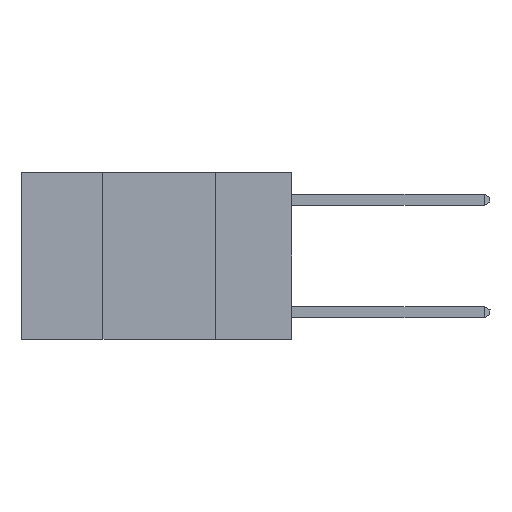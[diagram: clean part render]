
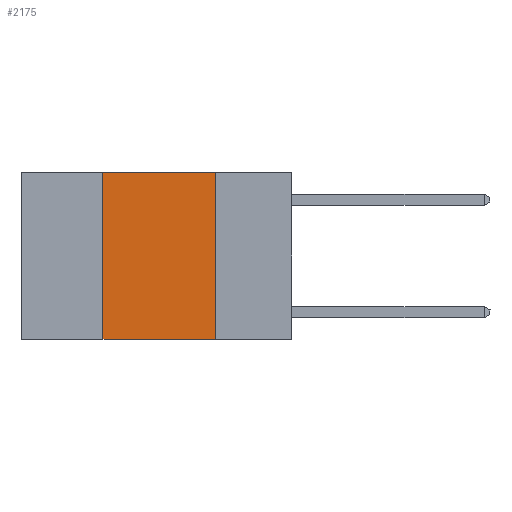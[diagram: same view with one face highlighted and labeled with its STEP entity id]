
A CAD part, left-side view. The second image highlights one B-rep face of the part: STEP entity #2175.
In plain terms, the highlighted planar face has unit normal (-1, 0, 0).
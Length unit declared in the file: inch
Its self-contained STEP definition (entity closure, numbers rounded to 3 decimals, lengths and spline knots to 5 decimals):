
#514 = PLANE ( 'NONE',  #21172 ) ;
#680 = VECTOR ( 'NONE', #9223, 39.37008 ) ;
#958 = EDGE_CURVE ( 'NONE', #5045, #11578, #18052, .T. ) ;
#1013 = CARTESIAN_POINT ( 'NONE',  ( 0., 0.42, -0.37 ) ) ;
#1327 = CARTESIAN_POINT ( 'NONE',  ( 0., 0.42, 0. ) ) ;
#2175 = ADVANCED_FACE ( 'NONE', ( #11949 ), #514, .F. ) ;
#2869 = VERTEX_POINT ( 'NONE', #16237 ) ;
#3985 = VECTOR ( 'NONE', #14567, 39.37008 ) ;
#4323 = LINE ( 'NONE', #11015, #21693 ) ;
#5045 = VERTEX_POINT ( 'NONE', #1327 ) ;
#5198 = EDGE_LOOP ( 'NONE', ( #8654, #17089, #20630, #5902 ) ) ;
#5756 = CARTESIAN_POINT ( 'NONE',  ( 0., 0.6, 0. ) ) ;
#5902 = ORIENTED_EDGE ( 'NONE', *, *, #13012, .T. ) ;
#7108 = VECTOR ( 'NONE', #20715, 39.37008 ) ;
#7189 = CARTESIAN_POINT ( 'NONE',  ( 0., 0.17, 0. ) ) ;
#8654 = ORIENTED_EDGE ( 'NONE', *, *, #18609, .F. ) ;
#9205 = DIRECTION ( 'NONE',  ( 0., 0., -1. ) ) ;
#9223 = DIRECTION ( 'NONE',  ( 0., 0., -1. ) ) ;
#11015 = CARTESIAN_POINT ( 'NONE',  ( 0., 0.42, 0. ) ) ;
#11111 = LINE ( 'NONE', #14100, #7108 ) ;
#11578 = VERTEX_POINT ( 'NONE', #7189 ) ;
#11949 = FACE_OUTER_BOUND ( 'NONE', #5198, .T. ) ;
#12713 = DIRECTION ( 'NONE',  ( 0., 0., 1. ) ) ;
#13012 = EDGE_CURVE ( 'NONE', #15362, #2869, #11111, .T. ) ;
#14100 = CARTESIAN_POINT ( 'NONE',  ( 0., 0.6, -0.37 ) ) ;
#14327 = LINE ( 'NONE', #19277, #680 ) ;
#14567 = DIRECTION ( 'NONE',  ( 0., -1., 0. ) ) ;
#15220 = EDGE_CURVE ( 'NONE', #15362, #5045, #4323, .T. ) ;
#15362 = VERTEX_POINT ( 'NONE', #1013 ) ;
#16237 = CARTESIAN_POINT ( 'NONE',  ( 0., 0.17, -0.37 ) ) ;
#17089 = ORIENTED_EDGE ( 'NONE', *, *, #958, .F. ) ;
#18052 = LINE ( 'NONE', #21232, #3985 ) ;
#18609 = EDGE_CURVE ( 'NONE', #11578, #2869, #14327, .T. ) ;
#19258 = DIRECTION ( 'NONE',  ( 1., 0., 0. ) ) ;
#19277 = CARTESIAN_POINT ( 'NONE',  ( 0., 0.17, 0. ) ) ;
#20630 = ORIENTED_EDGE ( 'NONE', *, *, #15220, .F. ) ;
#20715 = DIRECTION ( 'NONE',  ( 0., -1., 0. ) ) ;
#21172 = AXIS2_PLACEMENT_3D ( 'NONE', #5756, #19258, #9205 ) ;
#21232 = CARTESIAN_POINT ( 'NONE',  ( 0., 0.6, 0. ) ) ;
#21693 = VECTOR ( 'NONE', #12713, 39.37008 ) ;
